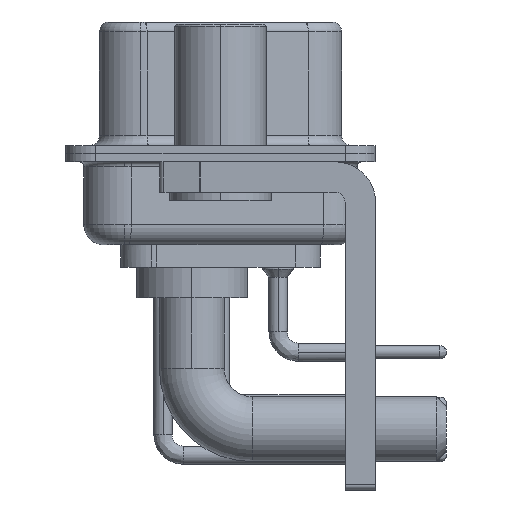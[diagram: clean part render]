
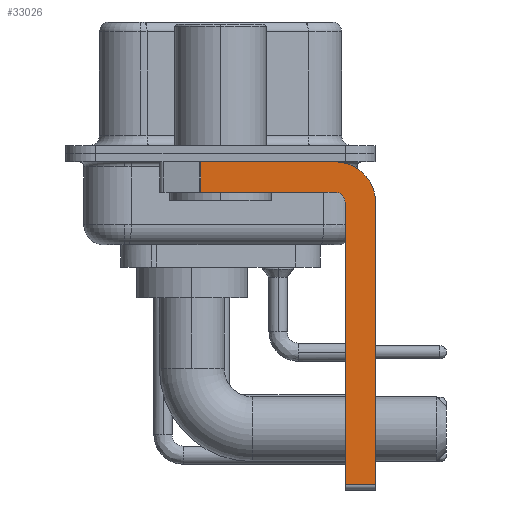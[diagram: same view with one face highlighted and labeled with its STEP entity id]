
A CAD part, left-side view. The second image highlights one B-rep face of the part: STEP entity #33026.
In plain terms, the highlighted planar face has unit normal (-1, 0, 0).
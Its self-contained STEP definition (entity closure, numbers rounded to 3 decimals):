
#562 = ORIENTED_EDGE ( 'NONE', *, *, #8134, .F. ) ;
#785 = CARTESIAN_POINT ( 'NONE',  ( -2.9, -5.65, -16.35 ) ) ;
#843 = EDGE_CURVE ( 'NONE', #29739, #27735, #30216, .T. ) ;
#1171 = PLANE ( 'NONE',  #11399 ) ;
#1247 = EDGE_CURVE ( 'NONE', #32673, #5638, #9863, .T. ) ;
#1404 = VECTOR ( 'NONE', #15682, 1000. ) ;
#1980 = LINE ( 'NONE', #4586, #11020 ) ;
#2230 = ORIENTED_EDGE ( 'NONE', *, *, #27314, .T. ) ;
#3255 = CARTESIAN_POINT ( 'NONE',  ( -2.9, -7.65, -2.4 ) ) ;
#4475 = VECTOR ( 'NONE', #19438, 1000. ) ;
#4586 = CARTESIAN_POINT ( 'NONE',  ( -2.9, -7.65, -2.4 ) ) ;
#4915 = DIRECTION ( 'NONE',  ( 1., 0., 0. ) ) ;
#5638 = VERTEX_POINT ( 'NONE', #3255 ) ;
#6761 = AXIS2_PLACEMENT_3D ( 'NONE', #24211, #27347, #35552 ) ;
#7306 = LINE ( 'NONE', #35180, #1404 ) ;
#7928 = CARTESIAN_POINT ( 'NONE',  ( -2.9, -5.65, -1.9 ) ) ;
#8134 = EDGE_CURVE ( 'NONE', #17522, #31759, #7306, .T. ) ;
#8221 = EDGE_CURVE ( 'NONE', #31759, #29739, #34035, .T. ) ;
#8477 = CARTESIAN_POINT ( 'NONE',  ( -2.9, 3., -0.4 ) ) ;
#8728 = CARTESIAN_POINT ( 'NONE',  ( -2.9, 0.978, -1.9 ) ) ;
#9726 = CARTESIAN_POINT ( 'NONE',  ( -2.9, -5.65, -2.4 ) ) ;
#9863 = CIRCLE ( 'NONE', #22284, 2. ) ;
#10328 = EDGE_CURVE ( 'NONE', #5638, #33299, #1980, .T. ) ;
#10667 = ORIENTED_EDGE ( 'NONE', *, *, #24935, .T. ) ;
#11020 = VECTOR ( 'NONE', #15936, 1000. ) ;
#11399 = AXIS2_PLACEMENT_3D ( 'NONE', #9726, #32544, #18259 ) ;
#11936 = CARTESIAN_POINT ( 'NONE',  ( -2.9, 0.978, -1.9 ) ) ;
#12768 = EDGE_CURVE ( 'NONE', #36129, #32673, #31684, .T. ) ;
#13984 = LINE ( 'NONE', #785, #33121 ) ;
#14058 = DIRECTION ( 'NONE',  ( 0., -1., 0. ) ) ;
#14336 = ORIENTED_EDGE ( 'NONE', *, *, #8221, .F. ) ;
#15086 = DIRECTION ( 'NONE',  ( 0., 0., -1. ) ) ;
#15682 = DIRECTION ( 'NONE',  ( 0., 0., 1. ) ) ;
#15936 = DIRECTION ( 'NONE',  ( 0., 0., -1. ) ) ;
#16436 = CARTESIAN_POINT ( 'NONE',  ( -2.9, -6.15, -2.4 ) ) ;
#16950 = CARTESIAN_POINT ( 'NONE',  ( -2.9, -7.65, -16.35 ) ) ;
#17522 = VERTEX_POINT ( 'NONE', #28457 ) ;
#18259 = DIRECTION ( 'NONE',  ( 0., 0., -1. ) ) ;
#19209 = CARTESIAN_POINT ( 'NONE',  ( -2.9, -5.65, -0.4 ) ) ;
#19438 = DIRECTION ( 'NONE',  ( 0., 1., 0. ) ) ;
#19506 = CARTESIAN_POINT ( 'NONE',  ( -2.9, 0.978, -0.4 ) ) ;
#21111 = ORIENTED_EDGE ( 'NONE', *, *, #12768, .F. ) ;
#22284 = AXIS2_PLACEMENT_3D ( 'NONE', #30352, #4915, #24246 ) ;
#24211 = CARTESIAN_POINT ( 'NONE',  ( -2.9, -5.65, -2.4 ) ) ;
#24246 = DIRECTION ( 'NONE',  ( 0., 0., -1. ) ) ;
#24935 = EDGE_CURVE ( 'NONE', #36129, #27735, #26590, .T. ) ;
#25325 = EDGE_LOOP ( 'NONE', ( #21111, #10667, #29063, #14336, #562, #2230, #35659, #29742 ) ) ;
#26583 = VECTOR ( 'NONE', #14058, 1000. ) ;
#26590 = LINE ( 'NONE', #11936, #35928 ) ;
#26616 = FACE_OUTER_BOUND ( 'NONE', #25325, .T. ) ;
#27314 = EDGE_CURVE ( 'NONE', #17522, #33299, #13984, .T. ) ;
#27347 = DIRECTION ( 'NONE',  ( -1., 0., 0. ) ) ;
#27735 = VERTEX_POINT ( 'NONE', #8728 ) ;
#28457 = CARTESIAN_POINT ( 'NONE',  ( -2.9, -6.15, -16.35 ) ) ;
#29063 = ORIENTED_EDGE ( 'NONE', *, *, #843, .F. ) ;
#29739 = VERTEX_POINT ( 'NONE', #35938 ) ;
#29742 = ORIENTED_EDGE ( 'NONE', *, *, #1247, .F. ) ;
#30216 = LINE ( 'NONE', #7928, #4475 ) ;
#30352 = CARTESIAN_POINT ( 'NONE',  ( -2.9, -5.65, -2.4 ) ) ;
#31684 = LINE ( 'NONE', #8477, #26583 ) ;
#31759 = VERTEX_POINT ( 'NONE', #16436 ) ;
#32544 = DIRECTION ( 'NONE',  ( 1., 0., 0. ) ) ;
#32673 = VERTEX_POINT ( 'NONE', #19209 ) ;
#33026 = ADVANCED_FACE ( 'NONE', ( #26616 ), #1171, .F. ) ;
#33121 = VECTOR ( 'NONE', #34223, 1000. ) ;
#33299 = VERTEX_POINT ( 'NONE', #16950 ) ;
#34035 = CIRCLE ( 'NONE', #6761, 0.5 ) ;
#34223 = DIRECTION ( 'NONE',  ( 0., -1., 0. ) ) ;
#35180 = CARTESIAN_POINT ( 'NONE',  ( -2.9, -6.15, -16.6 ) ) ;
#35552 = DIRECTION ( 'NONE',  ( 0., 0., 1. ) ) ;
#35659 = ORIENTED_EDGE ( 'NONE', *, *, #10328, .F. ) ;
#35928 = VECTOR ( 'NONE', #15086, 1000. ) ;
#35938 = CARTESIAN_POINT ( 'NONE',  ( -2.9, -5.65, -1.9 ) ) ;
#36129 = VERTEX_POINT ( 'NONE', #19506 ) ;
